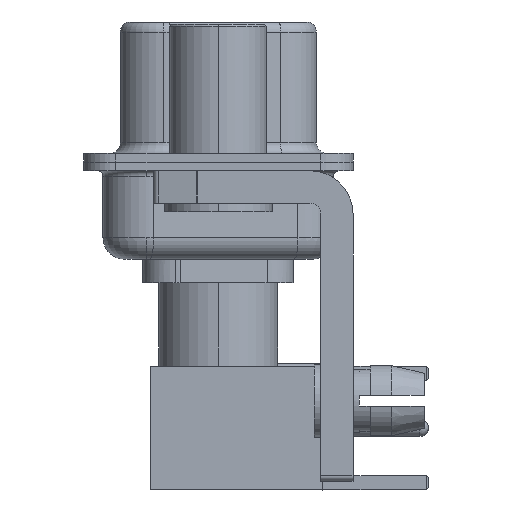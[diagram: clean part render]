
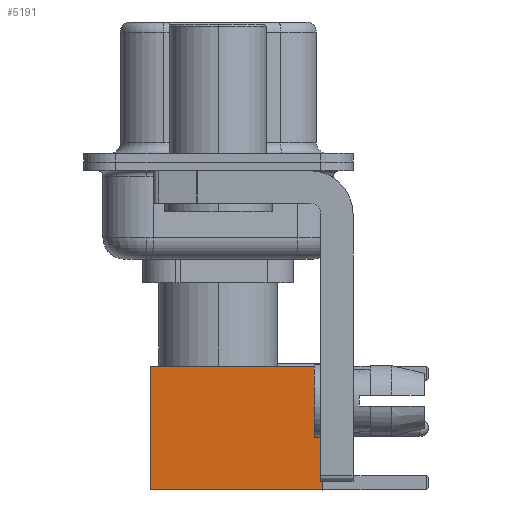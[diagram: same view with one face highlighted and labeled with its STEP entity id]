
A CAD part, left-side view. The second image highlights one B-rep face of the part: STEP entity #5191.
In plain terms, the highlighted face is planar.
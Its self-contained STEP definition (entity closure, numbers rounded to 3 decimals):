
#2165 = PLANE ( 'NONE',  #24306 ) ;
#5191 = ADVANCED_FACE ( 'NONE', ( #18674 ), #2165, .T. ) ;
#6639 = VERTEX_POINT ( 'NONE', #27762 ) ;
#6927 = VECTOR ( 'NONE', #33451, 1000. ) ;
#7122 = DIRECTION ( 'NONE',  ( 0., 0., -1. ) ) ;
#7810 = VECTOR ( 'NONE', #15988, 1000. ) ;
#11893 = ORIENTED_EDGE ( 'NONE', *, *, #30887, .F. ) ;
#12007 = CARTESIAN_POINT ( 'NONE',  ( -2.875, 2.875, 0. ) ) ;
#13267 = CARTESIAN_POINT ( 'NONE',  ( 0., 2.875, 8. ) ) ;
#13790 = EDGE_LOOP ( 'NONE', ( #20337, #22730, #26951, #11893 ) ) ;
#15065 = VERTEX_POINT ( 'NONE', #27151 ) ;
#15281 = LINE ( 'NONE', #12007, #31208 ) ;
#15682 = EDGE_CURVE ( 'NONE', #6639, #15065, #15281, .T. ) ;
#15742 = CARTESIAN_POINT ( 'NONE',  ( 2.875, 2.875, 0. ) ) ;
#15988 = DIRECTION ( 'NONE',  ( -1., 0., 0. ) ) ;
#16939 = LINE ( 'NONE', #22377, #6927 ) ;
#18674 = FACE_OUTER_BOUND ( 'NONE', #13790, .T. ) ;
#20337 = ORIENTED_EDGE ( 'NONE', *, *, #26799, .T. ) ;
#21221 = CARTESIAN_POINT ( 'NONE',  ( 2.875, 2.875, 0. ) ) ;
#21783 = LINE ( 'NONE', #13267, #7810 ) ;
#22069 = VERTEX_POINT ( 'NONE', #15742 ) ;
#22377 = CARTESIAN_POINT ( 'NONE',  ( 0., 2.875, 0. ) ) ;
#22730 = ORIENTED_EDGE ( 'NONE', *, *, #23764, .T. ) ;
#22779 = DIRECTION ( 'NONE',  ( 0., 0., -1. ) ) ;
#23764 = EDGE_CURVE ( 'NONE', #22069, #15065, #16939, .T. ) ;
#24306 = AXIS2_PLACEMENT_3D ( 'NONE', #21221, #26864, #27038 ) ;
#25327 = CARTESIAN_POINT ( 'NONE',  ( 2.875, 2.875, 0. ) ) ;
#25520 = VERTEX_POINT ( 'NONE', #31459 ) ;
#25523 = LINE ( 'NONE', #25327, #34944 ) ;
#26799 = EDGE_CURVE ( 'NONE', #25520, #22069, #25523, .T. ) ;
#26864 = DIRECTION ( 'NONE',  ( 0., 1., 0. ) ) ;
#26951 = ORIENTED_EDGE ( 'NONE', *, *, #15682, .F. ) ;
#27038 = DIRECTION ( 'NONE',  ( 0., 0., 1. ) ) ;
#27151 = CARTESIAN_POINT ( 'NONE',  ( -2.875, 2.875, 0. ) ) ;
#27762 = CARTESIAN_POINT ( 'NONE',  ( -2.875, 2.875, 8. ) ) ;
#30887 = EDGE_CURVE ( 'NONE', #25520, #6639, #21783, .T. ) ;
#31208 = VECTOR ( 'NONE', #7122, 1000. ) ;
#31459 = CARTESIAN_POINT ( 'NONE',  ( 2.875, 2.875, 8. ) ) ;
#33451 = DIRECTION ( 'NONE',  ( -1., 0., 0. ) ) ;
#34944 = VECTOR ( 'NONE', #22779, 1000. ) ;
